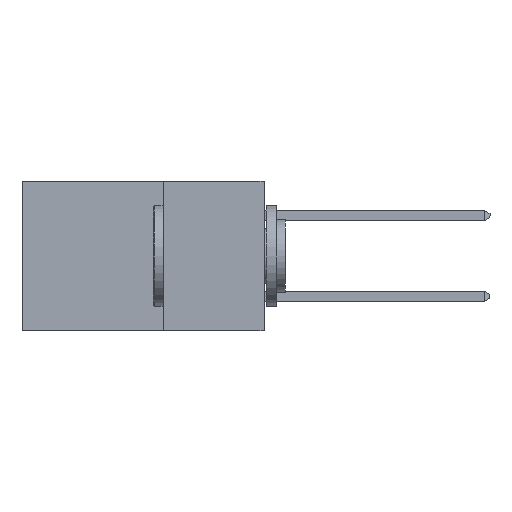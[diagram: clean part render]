
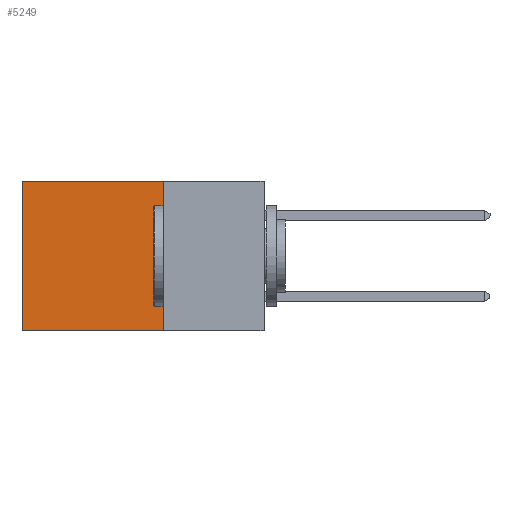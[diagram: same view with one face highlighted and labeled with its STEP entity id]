
A CAD part, left-side view. The second image highlights one B-rep face of the part: STEP entity #5249.
In plain terms, the highlighted planar face has unit normal (-1, 0, 0).
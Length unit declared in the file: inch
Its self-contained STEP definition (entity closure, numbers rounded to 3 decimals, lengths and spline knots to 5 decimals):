
#109 = VERTEX_POINT ( 'NONE', #9148 ) ;
#505 = EDGE_CURVE ( 'NONE', #9788, #4724, #1758, .T. ) ;
#694 = VECTOR ( 'NONE', #4015, 39.37008 ) ;
#1605 = DIRECTION ( 'NONE',  ( 1., 0., 0. ) ) ;
#1758 = LINE ( 'NONE', #3666, #2463 ) ;
#1995 = AXIS2_PLACEMENT_3D ( 'NONE', #5739, #1605, #8262 ) ;
#2273 = DIRECTION ( 'NONE',  ( 0., 1., 0. ) ) ;
#2424 = PLANE ( 'NONE',  #1995 ) ;
#2463 = VECTOR ( 'NONE', #5518, 39.37008 ) ;
#3146 = ORIENTED_EDGE ( 'NONE', *, *, #505, .F. ) ;
#3195 = CARTESIAN_POINT ( 'NONE',  ( 0.2615, 0.6, -0.37 ) ) ;
#3666 = CARTESIAN_POINT ( 'NONE',  ( 0.2615, 0.25, -0.37 ) ) ;
#3815 = LINE ( 'NONE', #9082, #694 ) ;
#4015 = DIRECTION ( 'NONE',  ( 0., 0., -1. ) ) ;
#4244 = CARTESIAN_POINT ( 'NONE',  ( 0.2615, 0.6, 0. ) ) ;
#4580 = VERTEX_POINT ( 'NONE', #4244 ) ;
#4724 = VERTEX_POINT ( 'NONE', #9544 ) ;
#5249 = ADVANCED_FACE ( 'NONE', ( #6559 ), #2424, .F. ) ;
#5337 = VECTOR ( 'NONE', #7404, 39.37008 ) ;
#5518 = DIRECTION ( 'NONE',  ( 0., 1., 0. ) ) ;
#5662 = VECTOR ( 'NONE', #2273, 39.37008 ) ;
#5739 = CARTESIAN_POINT ( 'NONE',  ( 0.2615, 0.25, -0.37 ) ) ;
#5848 = CARTESIAN_POINT ( 'NONE',  ( 0.2615, 0.25, -0.37 ) ) ;
#6259 = ORIENTED_EDGE ( 'NONE', *, *, #6372, .T. ) ;
#6372 = EDGE_CURVE ( 'NONE', #109, #4580, #9764, .T. ) ;
#6559 = FACE_OUTER_BOUND ( 'NONE', #9288, .T. ) ;
#6598 = ORIENTED_EDGE ( 'NONE', *, *, #9222, .F. ) ;
#7404 = DIRECTION ( 'NONE',  ( 0., 0., -1. ) ) ;
#8149 = EDGE_CURVE ( 'NONE', #4580, #4724, #10726, .T. ) ;
#8262 = DIRECTION ( 'NONE',  ( 0., 0., -1. ) ) ;
#9082 = CARTESIAN_POINT ( 'NONE',  ( 0.2615, 0.25, -0.37 ) ) ;
#9148 = CARTESIAN_POINT ( 'NONE',  ( 0.2615, 0.25, 0. ) ) ;
#9222 = EDGE_CURVE ( 'NONE', #109, #9788, #3815, .T. ) ;
#9288 = EDGE_LOOP ( 'NONE', ( #9766, #3146, #6598, #6259 ) ) ;
#9544 = CARTESIAN_POINT ( 'NONE',  ( 0.2615, 0.6, -0.37 ) ) ;
#9613 = CARTESIAN_POINT ( 'NONE',  ( 0.2615, 0.25, 0. ) ) ;
#9764 = LINE ( 'NONE', #9613, #5662 ) ;
#9766 = ORIENTED_EDGE ( 'NONE', *, *, #8149, .T. ) ;
#9788 = VERTEX_POINT ( 'NONE', #5848 ) ;
#10726 = LINE ( 'NONE', #3195, #5337 ) ;
